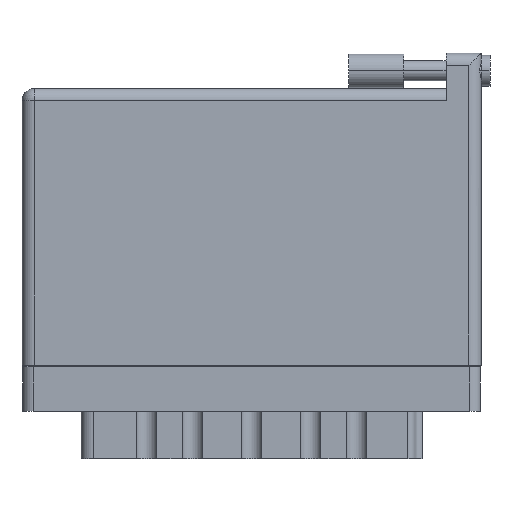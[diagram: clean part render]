
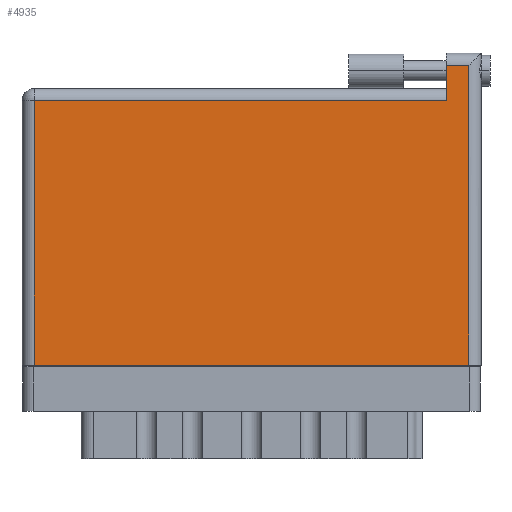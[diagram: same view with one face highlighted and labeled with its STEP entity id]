
A CAD part, front view. The second image highlights one B-rep face of the part: STEP entity #4935.
In plain terms, the highlighted face is planar.
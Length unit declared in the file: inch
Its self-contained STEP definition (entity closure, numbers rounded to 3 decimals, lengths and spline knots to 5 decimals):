
#341 = VERTEX_POINT ( 'NONE', #11604 ) ;
#660 = DIRECTION ( 'NONE',  ( -1., 0., 0. ) ) ;
#1501 = ORIENTED_EDGE ( 'NONE', *, *, #26196, .T. ) ;
#3596 = CARTESIAN_POINT ( 'NONE',  ( 0., 0., 0. ) ) ;
#4935 = ADVANCED_FACE ( 'NONE', ( #13203 ), #40637, .F. ) ;
#6169 = DIRECTION ( 'NONE',  ( -1., 0., 0. ) ) ;
#6410 = LINE ( 'NONE', #13646, #15796 ) ;
#7450 = VERTEX_POINT ( 'NONE', #41014 ) ;
#8356 = CARTESIAN_POINT ( 'NONE',  ( 0.07, 0., 0. ) ) ;
#10212 = DIRECTION ( 'NONE',  ( 0., 0., -1. ) ) ;
#11287 = LINE ( 'NONE', #33478, #36960 ) ;
#11604 = CARTESIAN_POINT ( 'NONE',  ( 2.403, 1.696, 0. ) ) ;
#12075 = VERTEX_POINT ( 'NONE', #8356 ) ;
#12442 = ORIENTED_EDGE ( 'NONE', *, *, #41990, .T. ) ;
#12597 = ORIENTED_EDGE ( 'NONE', *, *, #28189, .T. ) ;
#12745 = EDGE_CURVE ( 'NONE', #24550, #36398, #23738, .T. ) ;
#13203 = FACE_OUTER_BOUND ( 'NONE', #22353, .T. ) ;
#13646 = CARTESIAN_POINT ( 'NONE',  ( 0., 1.496, 0. ) ) ;
#13943 = CARTESIAN_POINT ( 'NONE',  ( 0., 1.566, 0. ) ) ;
#14568 = ORIENTED_EDGE ( 'NONE', *, *, #31163, .T. ) ;
#15374 = ORIENTED_EDGE ( 'NONE', *, *, #12745, .T. ) ;
#15796 = VECTOR ( 'NONE', #6169, 39.37008 ) ;
#17147 = ORIENTED_EDGE ( 'NONE', *, *, #22905, .T. ) ;
#18811 = DIRECTION ( 'NONE',  ( 1., 0., 0. ) ) ;
#20468 = VECTOR ( 'NONE', #18811, 39.37008 ) ;
#22353 = EDGE_LOOP ( 'NONE', ( #14568, #15374, #1501, #12597, #12442, #17147 ) ) ;
#22905 = EDGE_CURVE ( 'NONE', #41437, #12075, #30718, .T. ) ;
#23738 = LINE ( 'NONE', #28209, #29697 ) ;
#24550 = VERTEX_POINT ( 'NONE', #38167 ) ;
#26196 = EDGE_CURVE ( 'NONE', #36398, #341, #42332, .T. ) ;
#27222 = DIRECTION ( 'NONE',  ( 0., -1., 0. ) ) ;
#27707 = CARTESIAN_POINT ( 'NONE',  ( 0.07, 1.496, 0. ) ) ;
#28162 = VECTOR ( 'NONE', #660, 39.37008 ) ;
#28189 = EDGE_CURVE ( 'NONE', #341, #7450, #11287, .T. ) ;
#28209 = CARTESIAN_POINT ( 'NONE',  ( 2.53, 1.766, 0. ) ) ;
#29697 = VECTOR ( 'NONE', #31698, 39.37008 ) ;
#30718 = LINE ( 'NONE', #41960, #31095 ) ;
#31095 = VECTOR ( 'NONE', #27222, 39.37008 ) ;
#31163 = EDGE_CURVE ( 'NONE', #12075, #24550, #37772, .T. ) ;
#31698 = DIRECTION ( 'NONE',  ( 0., 1., 0. ) ) ;
#33478 = CARTESIAN_POINT ( 'NONE',  ( 2.403, 1.766, 0. ) ) ;
#36398 = VERTEX_POINT ( 'NONE', #43132 ) ;
#36651 = DIRECTION ( 'NONE',  ( -1., 0., 0. ) ) ;
#36960 = VECTOR ( 'NONE', #48729, 39.37008 ) ;
#37772 = LINE ( 'NONE', #3596, #20468 ) ;
#38167 = CARTESIAN_POINT ( 'NONE',  ( 2.53, 0., 0. ) ) ;
#40637 = PLANE ( 'NONE',  #41229 ) ;
#41014 = CARTESIAN_POINT ( 'NONE',  ( 2.403, 1.496, 0. ) ) ;
#41229 = AXIS2_PLACEMENT_3D ( 'NONE', #13943, #10212, #36651 ) ;
#41437 = VERTEX_POINT ( 'NONE', #27707 ) ;
#41960 = CARTESIAN_POINT ( 'NONE',  ( 0.07, 0., 0. ) ) ;
#41990 = EDGE_CURVE ( 'NONE', #7450, #41437, #6410, .T. ) ;
#42332 = LINE ( 'NONE', #46329, #28162 ) ;
#43132 = CARTESIAN_POINT ( 'NONE',  ( 2.53, 1.696, 0. ) ) ;
#46329 = CARTESIAN_POINT ( 'NONE',  ( 0., 1.696, 0. ) ) ;
#48729 = DIRECTION ( 'NONE',  ( 0., -1., 0. ) ) ;
